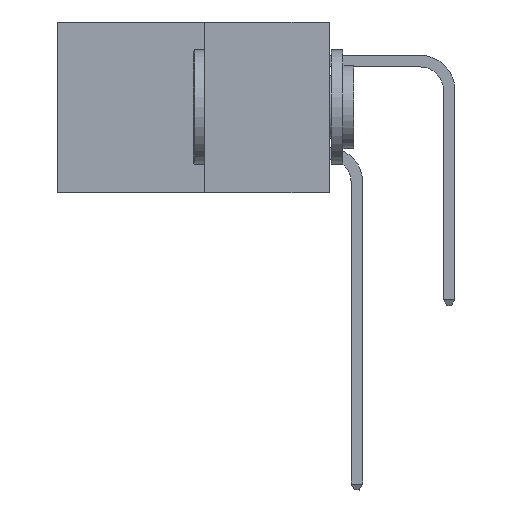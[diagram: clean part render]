
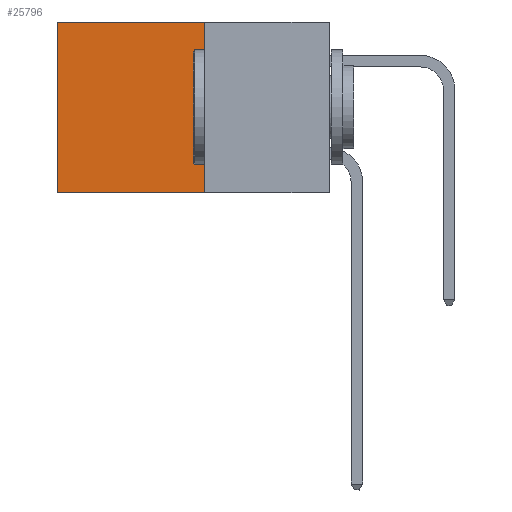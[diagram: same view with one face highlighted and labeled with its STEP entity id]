
A CAD part, left-side view. The second image highlights one B-rep face of the part: STEP entity #25796.
In plain terms, the highlighted planar face has unit normal (-1, 0, 0).
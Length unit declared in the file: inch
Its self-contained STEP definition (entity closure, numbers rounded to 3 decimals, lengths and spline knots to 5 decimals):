
#725 = VECTOR ( 'NONE', #22730, 39.37008 ) ;
#964 = VECTOR ( 'NONE', #3349, 39.37008 ) ;
#3349 = DIRECTION ( 'NONE',  ( 0., 0., -1. ) ) ;
#4398 = CARTESIAN_POINT ( 'NONE',  ( 0.277, 0.27, -0.37 ) ) ;
#4594 = ORIENTED_EDGE ( 'NONE', *, *, #26631, .F. ) ;
#4799 = CARTESIAN_POINT ( 'NONE',  ( 0.277, 0.27, -0.37 ) ) ;
#5686 = PLANE ( 'NONE',  #25799 ) ;
#6945 = CARTESIAN_POINT ( 'NONE',  ( 0.277, 0.59, 0. ) ) ;
#7031 = CARTESIAN_POINT ( 'NONE',  ( 0.277, 0.27, 0. ) ) ;
#8029 = VERTEX_POINT ( 'NONE', #6945 ) ;
#8044 = DIRECTION ( 'NONE',  ( 0., 0., -1. ) ) ;
#8129 = ORIENTED_EDGE ( 'NONE', *, *, #14926, .T. ) ;
#10153 = FACE_OUTER_BOUND ( 'NONE', #17678, .T. ) ;
#10328 = CARTESIAN_POINT ( 'NONE',  ( 0.277, 0.27, -0.37 ) ) ;
#13507 = LINE ( 'NONE', #4398, #25209 ) ;
#14926 = EDGE_CURVE ( 'NONE', #21114, #8029, #19620, .T. ) ;
#15218 = LINE ( 'NONE', #4799, #20740 ) ;
#16209 = ORIENTED_EDGE ( 'NONE', *, *, #20471, .F. ) ;
#16213 = VERTEX_POINT ( 'NONE', #25876 ) ;
#16233 = DIRECTION ( 'NONE',  ( 0., 1., 0. ) ) ;
#16479 = EDGE_CURVE ( 'NONE', #8029, #29303, #19855, .T. ) ;
#17678 = EDGE_LOOP ( 'NONE', ( #28427, #4594, #16209, #8129 ) ) ;
#19620 = LINE ( 'NONE', #20398, #725 ) ;
#19855 = LINE ( 'NONE', #19903, #964 ) ;
#19903 = CARTESIAN_POINT ( 'NONE',  ( 0.277, 0.59, -0.37 ) ) ;
#20398 = CARTESIAN_POINT ( 'NONE',  ( 0.277, 0.27, 0. ) ) ;
#20471 = EDGE_CURVE ( 'NONE', #21114, #16213, #15218, .T. ) ;
#20740 = VECTOR ( 'NONE', #28279, 39.37008 ) ;
#21114 = VERTEX_POINT ( 'NONE', #7031 ) ;
#22183 = DIRECTION ( 'NONE',  ( 1., 0., 0. ) ) ;
#22730 = DIRECTION ( 'NONE',  ( 0., 1., 0. ) ) ;
#25209 = VECTOR ( 'NONE', #16233, 39.37008 ) ;
#25796 = ADVANCED_FACE ( 'NONE', ( #10153 ), #5686, .F. ) ;
#25799 = AXIS2_PLACEMENT_3D ( 'NONE', #10328, #22183, #8044 ) ;
#25876 = CARTESIAN_POINT ( 'NONE',  ( 0.277, 0.27, -0.37 ) ) ;
#26631 = EDGE_CURVE ( 'NONE', #16213, #29303, #13507, .T. ) ;
#27669 = CARTESIAN_POINT ( 'NONE',  ( 0.277, 0.59, -0.37 ) ) ;
#28279 = DIRECTION ( 'NONE',  ( 0., 0., -1. ) ) ;
#28427 = ORIENTED_EDGE ( 'NONE', *, *, #16479, .T. ) ;
#29303 = VERTEX_POINT ( 'NONE', #27669 ) ;
